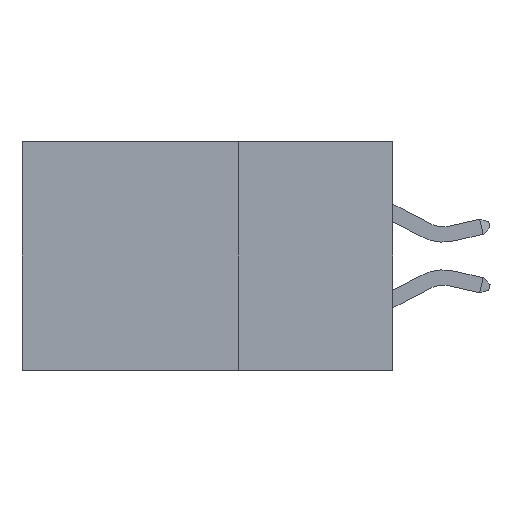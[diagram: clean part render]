
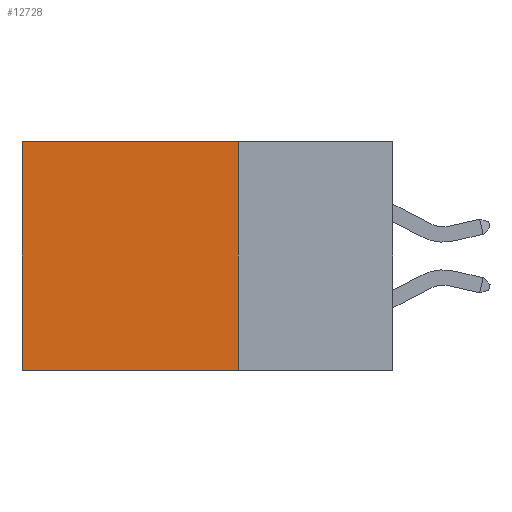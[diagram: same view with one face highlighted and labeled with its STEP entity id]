
A CAD part, left-side view. The second image highlights one B-rep face of the part: STEP entity #12728.
In plain terms, the highlighted planar face has unit normal (-1, 0, 0).
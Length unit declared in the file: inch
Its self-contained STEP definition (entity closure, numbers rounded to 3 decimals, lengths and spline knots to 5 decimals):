
#177 = CARTESIAN_POINT ( 'NONE',  ( 0.2875, 0.25, 0. ) ) ;
#272 = FACE_OUTER_BOUND ( 'NONE', #12206, .T. ) ;
#840 = ORIENTED_EDGE ( 'NONE', *, *, #1194, .T. ) ;
#915 = LINE ( 'NONE', #6477, #9945 ) ;
#1194 = EDGE_CURVE ( 'NONE', #11429, #9422, #7363, .T. ) ;
#2617 = DIRECTION ( 'NONE',  ( 0., 1., 0. ) ) ;
#3867 = LINE ( 'NONE', #20164, #15171 ) ;
#6467 = VERTEX_POINT ( 'NONE', #13401 ) ;
#6477 = CARTESIAN_POINT ( 'NONE',  ( 0.2875, 0.25, 0. ) ) ;
#6645 = CARTESIAN_POINT ( 'NONE',  ( 0.2875, 0.25, 0. ) ) ;
#7363 = LINE ( 'NONE', #6645, #7638 ) ;
#7638 = VECTOR ( 'NONE', #9099, 39.37008 ) ;
#8159 = AXIS2_PLACEMENT_3D ( 'NONE', #177, #17782, #16303 ) ;
#8436 = ORIENTED_EDGE ( 'NONE', *, *, #16207, .F. ) ;
#9099 = DIRECTION ( 'NONE',  ( 0., 1., 0. ) ) ;
#9422 = VERTEX_POINT ( 'NONE', #19843 ) ;
#9945 = VECTOR ( 'NONE', #17731, 39.37008 ) ;
#10063 = LINE ( 'NONE', #13739, #15590 ) ;
#10083 = EDGE_CURVE ( 'NONE', #9422, #6467, #3867, .T. ) ;
#11429 = VERTEX_POINT ( 'NONE', #13388 ) ;
#12162 = DIRECTION ( 'NONE',  ( 0., 0., -1. ) ) ;
#12206 = EDGE_LOOP ( 'NONE', ( #18812, #13907, #8436, #840 ) ) ;
#12728 = ADVANCED_FACE ( 'NONE', ( #272 ), #16374, .F. ) ;
#13388 = CARTESIAN_POINT ( 'NONE',  ( 0.2875, 0.25, 0. ) ) ;
#13401 = CARTESIAN_POINT ( 'NONE',  ( 0.2875, 0.6, -0.37 ) ) ;
#13739 = CARTESIAN_POINT ( 'NONE',  ( 0.2875, 0.25, -0.37 ) ) ;
#13907 = ORIENTED_EDGE ( 'NONE', *, *, #19723, .F. ) ;
#14163 = CARTESIAN_POINT ( 'NONE',  ( 0.2875, 0.25, -0.37 ) ) ;
#15171 = VECTOR ( 'NONE', #12162, 39.37008 ) ;
#15590 = VECTOR ( 'NONE', #2617, 39.37008 ) ;
#16207 = EDGE_CURVE ( 'NONE', #11429, #17219, #915, .T. ) ;
#16303 = DIRECTION ( 'NONE',  ( 0., 0., -1. ) ) ;
#16374 = PLANE ( 'NONE',  #8159 ) ;
#17219 = VERTEX_POINT ( 'NONE', #14163 ) ;
#17731 = DIRECTION ( 'NONE',  ( 0., 0., -1. ) ) ;
#17782 = DIRECTION ( 'NONE',  ( 1., 0., 0. ) ) ;
#18812 = ORIENTED_EDGE ( 'NONE', *, *, #10083, .T. ) ;
#19723 = EDGE_CURVE ( 'NONE', #17219, #6467, #10063, .T. ) ;
#19843 = CARTESIAN_POINT ( 'NONE',  ( 0.2875, 0.6, 0. ) ) ;
#20164 = CARTESIAN_POINT ( 'NONE',  ( 0.2875, 0.6, 0. ) ) ;
